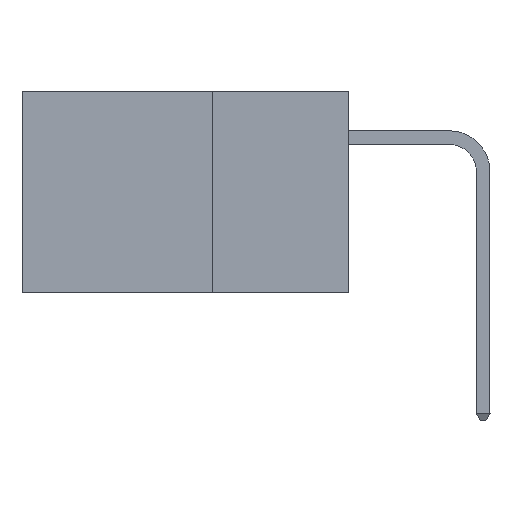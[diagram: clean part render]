
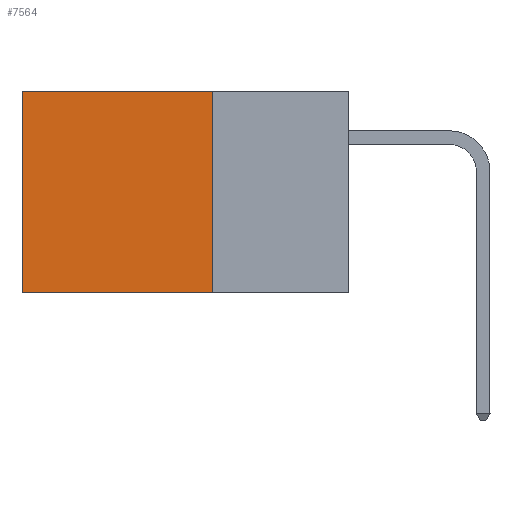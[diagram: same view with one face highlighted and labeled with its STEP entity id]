
A CAD part, left-side view. The second image highlights one B-rep face of the part: STEP entity #7564.
In plain terms, the highlighted planar face has unit normal (-1, 0, 0).
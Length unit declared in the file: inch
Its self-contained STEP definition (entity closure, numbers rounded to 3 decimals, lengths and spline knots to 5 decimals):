
#1580 = CARTESIAN_POINT ( 'NONE',  ( 0.2875, 0.25, -0.37 ) ) ;
#2144 = VECTOR ( 'NONE', #10740, 39.37008 ) ;
#2245 = DIRECTION ( 'NONE',  ( 0., 0., -1. ) ) ;
#2653 = CARTESIAN_POINT ( 'NONE',  ( 0.2875, 0.25, -0.37 ) ) ;
#3226 = CARTESIAN_POINT ( 'NONE',  ( 0.2875, 0.6, -0.37 ) ) ;
#3277 = FACE_OUTER_BOUND ( 'NONE', #13272, .T. ) ;
#3303 = VECTOR ( 'NONE', #6448, 39.37008 ) ;
#3656 = PLANE ( 'NONE',  #21500 ) ;
#4300 = LINE ( 'NONE', #15610, #18649 ) ;
#4742 = DIRECTION ( 'NONE',  ( 0., 0., -1. ) ) ;
#5740 = ORIENTED_EDGE ( 'NONE', *, *, #7749, .F. ) ;
#6448 = DIRECTION ( 'NONE',  ( 0., 0., -1. ) ) ;
#6994 = VECTOR ( 'NONE', #18373, 39.37008 ) ;
#7564 = ADVANCED_FACE ( 'NONE', ( #3277 ), #3656, .F. ) ;
#7749 = EDGE_CURVE ( 'NONE', #13758, #19023, #4300, .T. ) ;
#8749 = CARTESIAN_POINT ( 'NONE',  ( 0.2875, 0.25, 0. ) ) ;
#9772 = VERTEX_POINT ( 'NONE', #3226 ) ;
#10553 = LINE ( 'NONE', #8749, #6994 ) ;
#10740 = DIRECTION ( 'NONE',  ( 0., 1., 0. ) ) ;
#11685 = ORIENTED_EDGE ( 'NONE', *, *, #21512, .F. ) ;
#12471 = LINE ( 'NONE', #14284, #3303 ) ;
#13272 = EDGE_LOOP ( 'NONE', ( #13378, #11685, #5740, #21762 ) ) ;
#13378 = ORIENTED_EDGE ( 'NONE', *, *, #17551, .T. ) ;
#13758 = VERTEX_POINT ( 'NONE', #15117 ) ;
#14284 = CARTESIAN_POINT ( 'NONE',  ( 0.2875, 0.6, 0. ) ) ;
#15117 = CARTESIAN_POINT ( 'NONE',  ( 0.2875, 0.25, 0. ) ) ;
#15610 = CARTESIAN_POINT ( 'NONE',  ( 0.2875, 0.25, 0. ) ) ;
#17551 = EDGE_CURVE ( 'NONE', #19485, #9772, #12471, .T. ) ;
#18373 = DIRECTION ( 'NONE',  ( 0., 1., 0. ) ) ;
#18649 = VECTOR ( 'NONE', #2245, 39.37008 ) ;
#19023 = VERTEX_POINT ( 'NONE', #1580 ) ;
#19290 = EDGE_CURVE ( 'NONE', #13758, #19485, #10553, .T. ) ;
#19485 = VERTEX_POINT ( 'NONE', #24877 ) ;
#20229 = LINE ( 'NONE', #2653, #2144 ) ;
#20396 = CARTESIAN_POINT ( 'NONE',  ( 0.2875, 0.25, 0. ) ) ;
#21500 = AXIS2_PLACEMENT_3D ( 'NONE', #20396, #24236, #4742 ) ;
#21512 = EDGE_CURVE ( 'NONE', #19023, #9772, #20229, .T. ) ;
#21762 = ORIENTED_EDGE ( 'NONE', *, *, #19290, .T. ) ;
#24236 = DIRECTION ( 'NONE',  ( 1., 0., 0. ) ) ;
#24877 = CARTESIAN_POINT ( 'NONE',  ( 0.2875, 0.6, 0. ) ) ;
